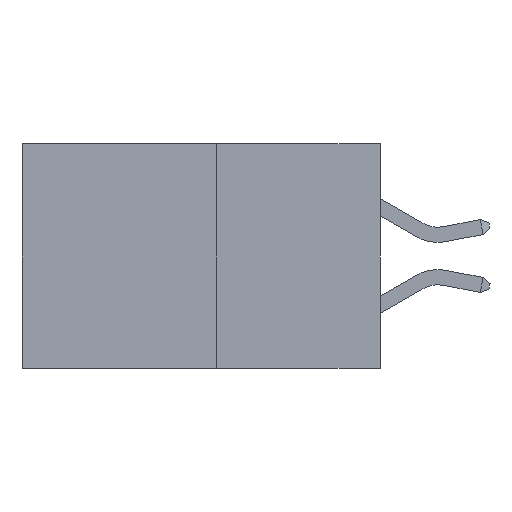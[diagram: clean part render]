
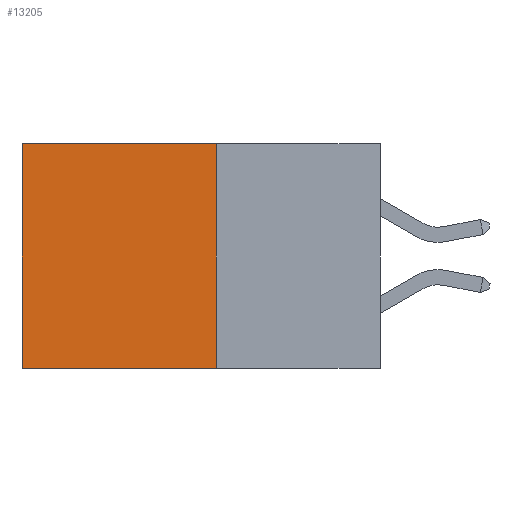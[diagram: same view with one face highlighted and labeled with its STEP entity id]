
A CAD part, left-side view. The second image highlights one B-rep face of the part: STEP entity #13205.
In plain terms, the highlighted planar face has unit normal (-1, 0, 0).
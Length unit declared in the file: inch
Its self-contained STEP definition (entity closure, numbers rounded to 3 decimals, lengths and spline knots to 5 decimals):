
#1612 = FACE_OUTER_BOUND ( 'NONE', #7010, .T. ) ;
#1755 = DIRECTION ( 'NONE',  ( 0., 0., -1. ) ) ;
#2172 = ORIENTED_EDGE ( 'NONE', *, *, #10358, .T. ) ;
#2587 = ORIENTED_EDGE ( 'NONE', *, *, #22285, .T. ) ;
#2984 = DIRECTION ( 'NONE',  ( 0., 1., 0. ) ) ;
#3496 = ORIENTED_EDGE ( 'NONE', *, *, #33495, .F. ) ;
#4060 = VERTEX_POINT ( 'NONE', #26597 ) ;
#5160 = ORIENTED_EDGE ( 'NONE', *, *, #23493, .F. ) ;
#5491 = VECTOR ( 'NONE', #34342, 39.37008 ) ;
#5739 = DIRECTION ( 'NONE',  ( 0., 0., -1. ) ) ;
#5995 = CARTESIAN_POINT ( 'NONE',  ( 0.277, 0.27, -0.37 ) ) ;
#6612 = CARTESIAN_POINT ( 'NONE',  ( 0.277, 0.59, 0. ) ) ;
#7010 = EDGE_LOOP ( 'NONE', ( #2587, #5160, #3496, #2172 ) ) ;
#7870 = VERTEX_POINT ( 'NONE', #27106 ) ;
#10358 = EDGE_CURVE ( 'NONE', #7870, #13764, #26452, .T. ) ;
#10994 = VERTEX_POINT ( 'NONE', #5995 ) ;
#11222 = CARTESIAN_POINT ( 'NONE',  ( 0.277, 0.27, 0. ) ) ;
#12970 = CARTESIAN_POINT ( 'NONE',  ( 0.277, 0.59, -0.37 ) ) ;
#13205 = ADVANCED_FACE ( 'NONE', ( #1612 ), #34118, .F. ) ;
#13764 = VERTEX_POINT ( 'NONE', #6612 ) ;
#13815 = VECTOR ( 'NONE', #5739, 39.37008 ) ;
#18124 = DIRECTION ( 'NONE',  ( 1., 0., 0. ) ) ;
#19277 = VECTOR ( 'NONE', #2984, 39.37008 ) ;
#22285 = EDGE_CURVE ( 'NONE', #13764, #4060, #27910, .T. ) ;
#23493 = EDGE_CURVE ( 'NONE', #10994, #4060, #31124, .T. ) ;
#24827 = CARTESIAN_POINT ( 'NONE',  ( 0.277, 0.27, -0.37 ) ) ;
#26452 = LINE ( 'NONE', #11222, #19277 ) ;
#26597 = CARTESIAN_POINT ( 'NONE',  ( 0.277, 0.59, -0.37 ) ) ;
#27106 = CARTESIAN_POINT ( 'NONE',  ( 0.277, 0.27, 0. ) ) ;
#27910 = LINE ( 'NONE', #12970, #5491 ) ;
#28886 = LINE ( 'NONE', #29912, #13815 ) ;
#29912 = CARTESIAN_POINT ( 'NONE',  ( 0.277, 0.27, -0.37 ) ) ;
#30018 = DIRECTION ( 'NONE',  ( 0., 1., 0. ) ) ;
#30289 = VECTOR ( 'NONE', #30018, 39.37008 ) ;
#31124 = LINE ( 'NONE', #24827, #30289 ) ;
#31463 = CARTESIAN_POINT ( 'NONE',  ( 0.277, 0.27, -0.37 ) ) ;
#33036 = AXIS2_PLACEMENT_3D ( 'NONE', #31463, #18124, #1755 ) ;
#33495 = EDGE_CURVE ( 'NONE', #7870, #10994, #28886, .T. ) ;
#34118 = PLANE ( 'NONE',  #33036 ) ;
#34342 = DIRECTION ( 'NONE',  ( 0., 0., -1. ) ) ;
